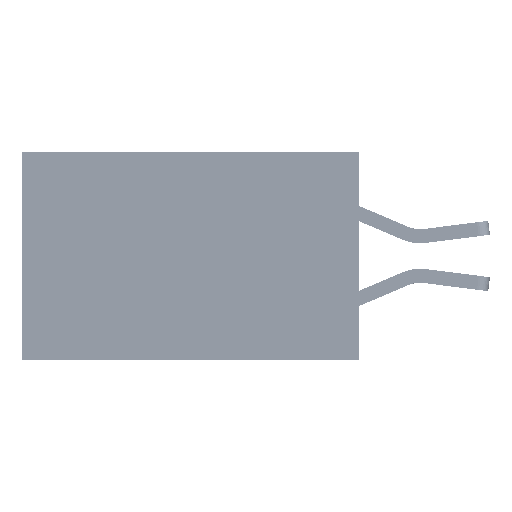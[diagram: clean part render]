
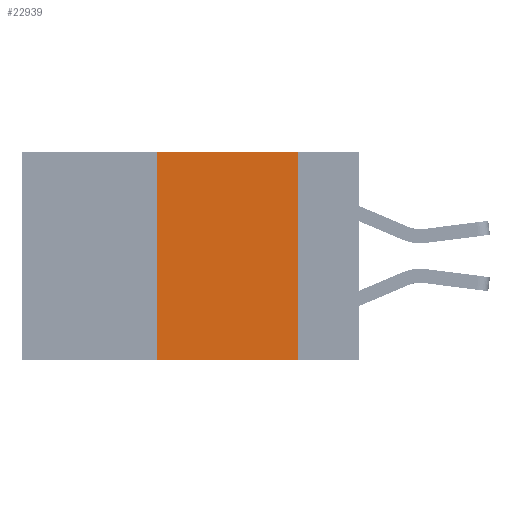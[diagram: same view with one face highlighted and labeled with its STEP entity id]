
A CAD part, left-side view. The second image highlights one B-rep face of the part: STEP entity #22939.
In plain terms, the highlighted planar face has unit normal (-1, 0, 0).
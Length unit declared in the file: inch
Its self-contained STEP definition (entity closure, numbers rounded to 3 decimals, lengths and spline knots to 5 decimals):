
#65 = CARTESIAN_POINT ( 'NONE',  ( 0., 0.36, 0. ) ) ;
#1235 = CARTESIAN_POINT ( 'NONE',  ( 0., 0.6, 0. ) ) ;
#2060 = FACE_OUTER_BOUND ( 'NONE', #2510, .T. ) ;
#2510 = EDGE_LOOP ( 'NONE', ( #20544, #2620, #8684, #18949 ) ) ;
#2620 = ORIENTED_EDGE ( 'NONE', *, *, #25500, .F. ) ;
#4564 = CARTESIAN_POINT ( 'NONE',  ( 0., 0.6, 0. ) ) ;
#4816 = CARTESIAN_POINT ( 'NONE',  ( 0., 0.6, -0.37 ) ) ;
#4960 = DIRECTION ( 'NONE',  ( 1., 0., 0. ) ) ;
#7385 = DIRECTION ( 'NONE',  ( 0., -1., 0. ) ) ;
#7913 = DIRECTION ( 'NONE',  ( 0., 0., -1. ) ) ;
#8068 = VECTOR ( 'NONE', #25522, 39.37008 ) ;
#8684 = ORIENTED_EDGE ( 'NONE', *, *, #31303, .F. ) ;
#11318 = LINE ( 'NONE', #65, #12270 ) ;
#12270 = VECTOR ( 'NONE', #27087, 39.37008 ) ;
#13816 = VERTEX_POINT ( 'NONE', #31530 ) ;
#15753 = VERTEX_POINT ( 'NONE', #20733 ) ;
#17684 = VECTOR ( 'NONE', #30822, 39.37008 ) ;
#18949 = ORIENTED_EDGE ( 'NONE', *, *, #22864, .T. ) ;
#20544 = ORIENTED_EDGE ( 'NONE', *, *, #31384, .F. ) ;
#20733 = CARTESIAN_POINT ( 'NONE',  ( 0., 0.36, -0.37 ) ) ;
#22451 = CARTESIAN_POINT ( 'NONE',  ( 0., 0.11, -0.37 ) ) ;
#22864 = EDGE_CURVE ( 'NONE', #15753, #24191, #23619, .T. ) ;
#22939 = ADVANCED_FACE ( 'NONE', ( #2060 ), #27901, .F. ) ;
#23619 = LINE ( 'NONE', #4816, #17684 ) ;
#24035 = CARTESIAN_POINT ( 'NONE',  ( 0., 0.36, 0. ) ) ;
#24191 = VERTEX_POINT ( 'NONE', #22451 ) ;
#25500 = EDGE_CURVE ( 'NONE', #34605, #13816, #28872, .T. ) ;
#25522 = DIRECTION ( 'NONE',  ( 0., 0., -1. ) ) ;
#27087 = DIRECTION ( 'NONE',  ( 0., 0., 1. ) ) ;
#27901 = PLANE ( 'NONE',  #31863 ) ;
#28872 = LINE ( 'NONE', #1235, #30698 ) ;
#29600 = LINE ( 'NONE', #31377, #8068 ) ;
#30698 = VECTOR ( 'NONE', #7385, 39.37008 ) ;
#30822 = DIRECTION ( 'NONE',  ( 0., -1., 0. ) ) ;
#31303 = EDGE_CURVE ( 'NONE', #15753, #34605, #11318, .T. ) ;
#31377 = CARTESIAN_POINT ( 'NONE',  ( 0., 0.11, 0. ) ) ;
#31384 = EDGE_CURVE ( 'NONE', #13816, #24191, #29600, .T. ) ;
#31530 = CARTESIAN_POINT ( 'NONE',  ( 0., 0.11, 0. ) ) ;
#31863 = AXIS2_PLACEMENT_3D ( 'NONE', #4564, #4960, #7913 ) ;
#34605 = VERTEX_POINT ( 'NONE', #24035 ) ;
